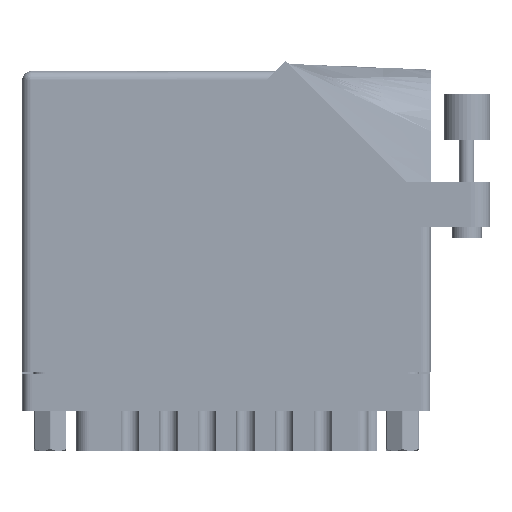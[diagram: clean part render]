
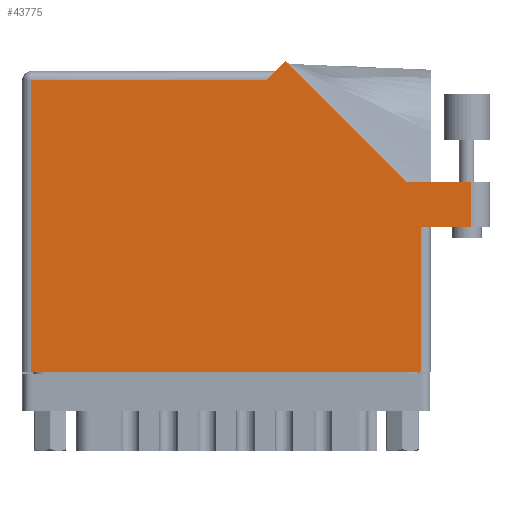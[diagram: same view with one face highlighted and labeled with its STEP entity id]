
A CAD part, front view. The second image highlights one B-rep face of the part: STEP entity #43775.
In plain terms, the highlighted face is planar.
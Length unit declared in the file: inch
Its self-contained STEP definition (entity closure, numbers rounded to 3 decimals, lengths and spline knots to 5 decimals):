
#935 = LINE ( 'NONE', #20010, #84277 ) ;
#3449 = CARTESIAN_POINT ( 'NONE',  ( 3.03, 1.287, 0. ) ) ;
#12995 = LINE ( 'NONE', #36925, #98877 ) ;
#14577 = DIRECTION ( 'NONE',  ( -1., 0., 0. ) ) ;
#14969 = LINE ( 'NONE', #93148, #61203 ) ;
#15576 = CARTESIAN_POINT ( 'NONE',  ( 2.693, 0., 0. ) ) ;
#17072 = LINE ( 'NONE', #17851, #54221 ) ;
#17851 = CARTESIAN_POINT ( 'NONE',  ( 2.693, 0.98, 0. ) ) ;
#17952 = VERTEX_POINT ( 'NONE', #3449 ) ;
#18276 = EDGE_CURVE ( 'NONE', #17952, #73219, #40701, .T. ) ;
#20010 = CARTESIAN_POINT ( 'NONE',  ( 3.03, 1.287, 0. ) ) ;
#22210 = CARTESIAN_POINT ( 'NONE',  ( 0.062, 0., 0. ) ) ;
#22862 = CARTESIAN_POINT ( 'NONE',  ( 2.755, 0.98, 0. ) ) ;
#25234 = DIRECTION ( 'NONE',  ( 0., 0., -1. ) ) ;
#25685 = CARTESIAN_POINT ( 'NONE',  ( 1.643, 1.968, 0. ) ) ;
#26320 = DIRECTION ( 'NONE',  ( -0.707, -0.707, 0. ) ) ;
#27103 = LINE ( 'NONE', #73479, #89979 ) ;
#27864 = DIRECTION ( 'NONE',  ( 0., -1., 0. ) ) ;
#28179 = EDGE_CURVE ( 'NONE', #88939, #87965, #17072, .T. ) ;
#28465 = ORIENTED_EDGE ( 'NONE', *, *, #72188, .T. ) ;
#33174 = LINE ( 'NONE', #22862, #62766 ) ;
#34149 = CARTESIAN_POINT ( 'NONE',  ( 2.58942, 1.287, 0. ) ) ;
#34884 = CARTESIAN_POINT ( 'NONE',  ( 3.155, 1.287, 0. ) ) ;
#35962 = VERTEX_POINT ( 'NONE', #61650 ) ;
#36925 = CARTESIAN_POINT ( 'NONE',  ( 2.58942, 1.287, 0. ) ) ;
#40701 = LINE ( 'NONE', #34884, #48398 ) ;
#40719 = PLANE ( 'NONE',  #55802 ) ;
#41894 = DIRECTION ( 'NONE',  ( 1., 0., 0. ) ) ;
#43775 = ADVANCED_FACE ( 'NONE', ( #78615 ), #40719, .F. ) ;
#44728 = DIRECTION ( 'NONE',  ( 0., 1., 0. ) ) ;
#46343 = ORIENTED_EDGE ( 'NONE', *, *, #59802, .T. ) ;
#46869 = VECTOR ( 'NONE', #14577, 39.37008 ) ;
#47057 = EDGE_CURVE ( 'NONE', #86560, #17952, #935, .T. ) ;
#48398 = VECTOR ( 'NONE', #92265, 39.37008 ) ;
#49658 = CARTESIAN_POINT ( 'NONE',  ( 0., 2.03, 0. ) ) ;
#50834 = EDGE_CURVE ( 'NONE', #74975, #88939, #27103, .T. ) ;
#54221 = VECTOR ( 'NONE', #98492, 39.37008 ) ;
#55802 = AXIS2_PLACEMENT_3D ( 'NONE', #49658, #25234, #82283 ) ;
#58284 = EDGE_CURVE ( 'NONE', #73219, #85154, #12995, .T. ) ;
#58611 = CARTESIAN_POINT ( 'NONE',  ( 1.705, 2.03, 0. ) ) ;
#59167 = ORIENTED_EDGE ( 'NONE', *, *, #58284, .T. ) ;
#59802 = EDGE_CURVE ( 'NONE', #85154, #61038, #103950, .T. ) ;
#60366 = VECTOR ( 'NONE', #26320, 39.37008 ) ;
#61038 = VERTEX_POINT ( 'NONE', #25685 ) ;
#61203 = VECTOR ( 'NONE', #27864, 39.37008 ) ;
#61255 = ORIENTED_EDGE ( 'NONE', *, *, #63899, .T. ) ;
#61650 = CARTESIAN_POINT ( 'NONE',  ( 0.062, 1.968, 0. ) ) ;
#62353 = LINE ( 'NONE', #65161, #46869 ) ;
#62766 = VECTOR ( 'NONE', #95307, 39.37008 ) ;
#63899 = EDGE_CURVE ( 'NONE', #35962, #74975, #14969, .T. ) ;
#65161 = CARTESIAN_POINT ( 'NONE',  ( 0., 1.968, 0. ) ) ;
#72188 = EDGE_CURVE ( 'NONE', #87965, #86560, #33174, .T. ) ;
#73076 = ORIENTED_EDGE ( 'NONE', *, *, #50834, .T. ) ;
#73128 = CARTESIAN_POINT ( 'NONE',  ( 3.03, 0.98, 0. ) ) ;
#73219 = VERTEX_POINT ( 'NONE', #34149 ) ;
#73479 = CARTESIAN_POINT ( 'NONE',  ( 0., 0., 0. ) ) ;
#74975 = VERTEX_POINT ( 'NONE', #22210 ) ;
#77430 = CARTESIAN_POINT ( 'NONE',  ( 1.77571, 2.10071, 0. ) ) ;
#77717 = ORIENTED_EDGE ( 'NONE', *, *, #18276, .T. ) ;
#78615 = FACE_OUTER_BOUND ( 'NONE', #96080, .T. ) ;
#82038 = EDGE_CURVE ( 'NONE', #61038, #35962, #62353, .T. ) ;
#82283 = DIRECTION ( 'NONE',  ( -1., 0., 0. ) ) ;
#84277 = VECTOR ( 'NONE', #44728, 39.37008 ) ;
#85007 = CARTESIAN_POINT ( 'NONE',  ( 2.693, 0.98, 0. ) ) ;
#85154 = VERTEX_POINT ( 'NONE', #77430 ) ;
#86560 = VERTEX_POINT ( 'NONE', #73128 ) ;
#87965 = VERTEX_POINT ( 'NONE', #85007 ) ;
#88939 = VERTEX_POINT ( 'NONE', #15576 ) ;
#89979 = VECTOR ( 'NONE', #41894, 39.37008 ) ;
#91864 = ORIENTED_EDGE ( 'NONE', *, *, #47057, .T. ) ;
#92265 = DIRECTION ( 'NONE',  ( -1., 0., 0. ) ) ;
#93148 = CARTESIAN_POINT ( 'NONE',  ( 0.062, 0., 0. ) ) ;
#93579 = DIRECTION ( 'NONE',  ( -0.707, 0.707, 0. ) ) ;
#95276 = ORIENTED_EDGE ( 'NONE', *, *, #28179, .T. ) ;
#95307 = DIRECTION ( 'NONE',  ( 1., 0., 0. ) ) ;
#96080 = EDGE_LOOP ( 'NONE', ( #28465, #91864, #77717, #59167, #46343, #106087, #61255, #73076, #95276 ) ) ;
#98492 = DIRECTION ( 'NONE',  ( 0., 1., 0. ) ) ;
#98877 = VECTOR ( 'NONE', #93579, 39.37008 ) ;
#103950 = LINE ( 'NONE', #58611, #60366 ) ;
#106087 = ORIENTED_EDGE ( 'NONE', *, *, #82038, .T. ) ;
